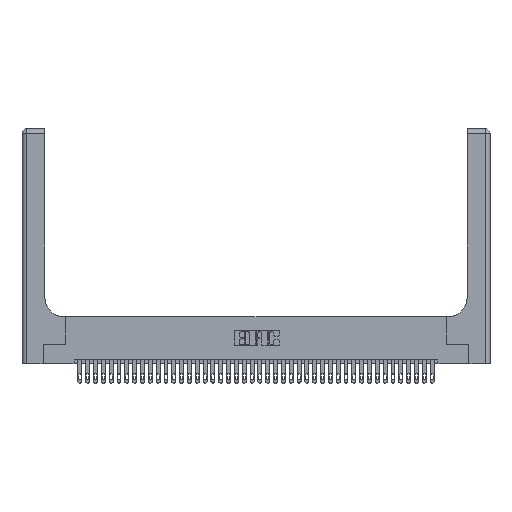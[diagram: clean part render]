
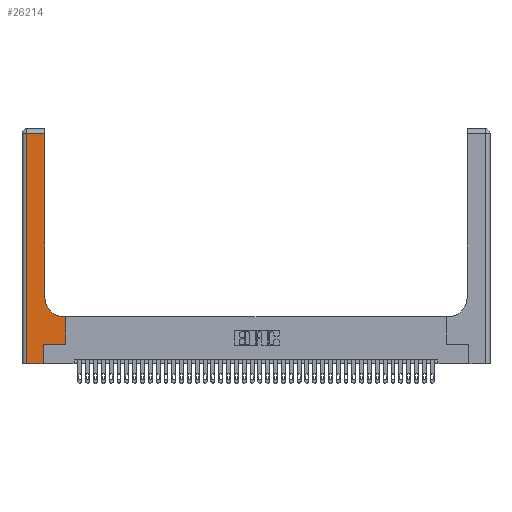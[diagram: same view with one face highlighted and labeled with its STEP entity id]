
A CAD part, top view. The second image highlights one B-rep face of the part: STEP entity #26214.
In plain terms, the highlighted planar face has unit normal (0, 0, 1).
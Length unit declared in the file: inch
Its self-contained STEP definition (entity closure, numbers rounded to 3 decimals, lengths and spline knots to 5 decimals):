
#99 = CARTESIAN_POINT ( 'NONE',  ( 0.5415, 0.6, 0.37 ) ) ;
#148 = CARTESIAN_POINT ( 'NONE',  ( 0.5585, 0.6, 0.37 ) ) ;
#897 = ORIENTED_EDGE ( 'NONE', *, *, #22168, .T. ) ;
#1011 = CARTESIAN_POINT ( 'NONE',  ( 0.2915, 3., 0.37 ) ) ;
#1164 = DIRECTION ( 'NONE',  ( 0., 1., 0. ) ) ;
#1583 = CARTESIAN_POINT ( 'NONE',  ( 0.06, 0., 0.37 ) ) ;
#1870 = DIRECTION ( 'NONE',  ( -1., 0., 0. ) ) ;
#4359 = CARTESIAN_POINT ( 'NONE',  ( 0., 2.94, 0.37 ) ) ;
#4771 = DIRECTION ( 'NONE',  ( 0., 0., -1. ) ) ;
#4780 = VERTEX_POINT ( 'NONE', #26808 ) ;
#5262 = FACE_OUTER_BOUND ( 'NONE', #19138, .T. ) ;
#5919 = VERTEX_POINT ( 'NONE', #26336 ) ;
#6045 = EDGE_CURVE ( 'NONE', #15525, #33211, #22997, .T. ) ;
#6441 = DIRECTION ( 'NONE',  ( 0., 1., 0. ) ) ;
#6550 = LINE ( 'NONE', #1011, #36106 ) ;
#6943 = LINE ( 'NONE', #34296, #8414 ) ;
#7186 = PLANE ( 'NONE',  #24144 ) ;
#8265 = DIRECTION ( 'NONE',  ( -1., 0., 0. ) ) ;
#8414 = VECTOR ( 'NONE', #34044, 39.37008 ) ;
#8607 = VECTOR ( 'NONE', #1870, 39.37008 ) ;
#8921 = EDGE_CURVE ( 'NONE', #23945, #5919, #11125, .T. ) ;
#9363 = LINE ( 'NONE', #4359, #30036 ) ;
#10311 = DIRECTION ( 'NONE',  ( 0., 0., -1. ) ) ;
#10724 = CARTESIAN_POINT ( 'NONE',  ( 0.06, 2.94, 0.37 ) ) ;
#10841 = ORIENTED_EDGE ( 'NONE', *, *, #21319, .T. ) ;
#11125 = CIRCLE ( 'NONE', #26904, 0.25 ) ;
#11726 = CARTESIAN_POINT ( 'NONE',  ( 0.269, 0.25, 0.37 ) ) ;
#12953 = EDGE_CURVE ( 'NONE', #15944, #15525, #6943, .T. ) ;
#13179 = DIRECTION ( 'NONE',  ( 0., 1., 0. ) ) ;
#13697 = EDGE_CURVE ( 'NONE', #4780, #16958, #9363, .T. ) ;
#13961 = ORIENTED_EDGE ( 'NONE', *, *, #6045, .T. ) ;
#14027 = DIRECTION ( 'NONE',  ( 0., -1., 0. ) ) ;
#14576 = ORIENTED_EDGE ( 'NONE', *, *, #19858, .T. ) ;
#15525 = VERTEX_POINT ( 'NONE', #25533 ) ;
#15860 = EDGE_CURVE ( 'NONE', #5919, #4780, #6550, .T. ) ;
#15944 = VERTEX_POINT ( 'NONE', #1583 ) ;
#16630 = CARTESIAN_POINT ( 'NONE',  ( 0.5415, 0.85, 0.37 ) ) ;
#16682 = ORIENTED_EDGE ( 'NONE', *, *, #15860, .T. ) ;
#16958 = VERTEX_POINT ( 'NONE', #10724 ) ;
#18213 = CARTESIAN_POINT ( 'NONE',  ( 0.269, 0., 0.37 ) ) ;
#18567 = VECTOR ( 'NONE', #14027, 39.37008 ) ;
#18889 = ORIENTED_EDGE ( 'NONE', *, *, #8921, .T. ) ;
#19138 = EDGE_LOOP ( 'NONE', ( #16682, #23842, #26573, #24629, #13961, #897, #14576, #10841, #18889 ) ) ;
#19855 = LINE ( 'NONE', #20713, #8607 ) ;
#19858 = EDGE_CURVE ( 'NONE', #26591, #36464, #20887, .T. ) ;
#20713 = CARTESIAN_POINT ( 'NONE',  ( 0.2915, 0.6, 0.37 ) ) ;
#20887 = LINE ( 'NONE', #28723, #39185 ) ;
#21319 = EDGE_CURVE ( 'NONE', #36464, #23945, #19855, .T. ) ;
#22029 = VECTOR ( 'NONE', #6441, 39.37008 ) ;
#22168 = EDGE_CURVE ( 'NONE', #33211, #26591, #40521, .T. ) ;
#22997 = LINE ( 'NONE', #18213, #22029 ) ;
#23427 = CARTESIAN_POINT ( 'NONE',  ( 0.269, 0.25, 0.37 ) ) ;
#23842 = ORIENTED_EDGE ( 'NONE', *, *, #13697, .T. ) ;
#23945 = VERTEX_POINT ( 'NONE', #99 ) ;
#24144 = AXIS2_PLACEMENT_3D ( 'NONE', #38989, #10311, #35517 ) ;
#24189 = VECTOR ( 'NONE', #24482, 39.37008 ) ;
#24482 = DIRECTION ( 'NONE',  ( 1., 0., 0. ) ) ;
#24629 = ORIENTED_EDGE ( 'NONE', *, *, #12953, .T. ) ;
#25533 = CARTESIAN_POINT ( 'NONE',  ( 0.269, 0., 0.37 ) ) ;
#26214 = ADVANCED_FACE ( 'NONE', ( #5262 ), #7186, .F. ) ;
#26336 = CARTESIAN_POINT ( 'NONE',  ( 0.2915, 0.85, 0.37 ) ) ;
#26573 = ORIENTED_EDGE ( 'NONE', *, *, #31235, .T. ) ;
#26591 = VERTEX_POINT ( 'NONE', #37825 ) ;
#26808 = CARTESIAN_POINT ( 'NONE',  ( 0.2915, 2.94, 0.37 ) ) ;
#26904 = AXIS2_PLACEMENT_3D ( 'NONE', #16630, #4771, #27060 ) ;
#27060 = DIRECTION ( 'NONE',  ( 1., 0., 0. ) ) ;
#28723 = CARTESIAN_POINT ( 'NONE',  ( 0.5585, 0.25, 0.37 ) ) ;
#29578 = CARTESIAN_POINT ( 'NONE',  ( 0.06, 3., 0.37 ) ) ;
#30036 = VECTOR ( 'NONE', #8265, 39.37008 ) ;
#31235 = EDGE_CURVE ( 'NONE', #16958, #15944, #39852, .T. ) ;
#33211 = VERTEX_POINT ( 'NONE', #23427 ) ;
#34044 = DIRECTION ( 'NONE',  ( 1., 0., 0. ) ) ;
#34296 = CARTESIAN_POINT ( 'NONE',  ( 0., 0., 0.37 ) ) ;
#35517 = DIRECTION ( 'NONE',  ( -1., 0., 0. ) ) ;
#36106 = VECTOR ( 'NONE', #1164, 39.37008 ) ;
#36464 = VERTEX_POINT ( 'NONE', #148 ) ;
#37825 = CARTESIAN_POINT ( 'NONE',  ( 0.5585, 0.25, 0.37 ) ) ;
#38989 = CARTESIAN_POINT ( 'NONE',  ( 0., 3., 0.37 ) ) ;
#39185 = VECTOR ( 'NONE', #13179, 39.37008 ) ;
#39852 = LINE ( 'NONE', #29578, #18567 ) ;
#40521 = LINE ( 'NONE', #11726, #24189 ) ;
